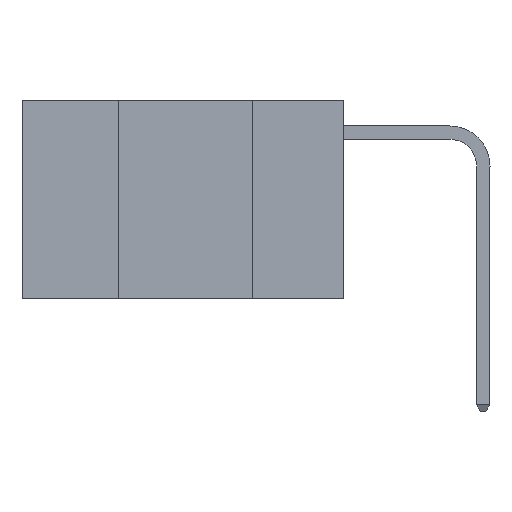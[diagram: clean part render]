
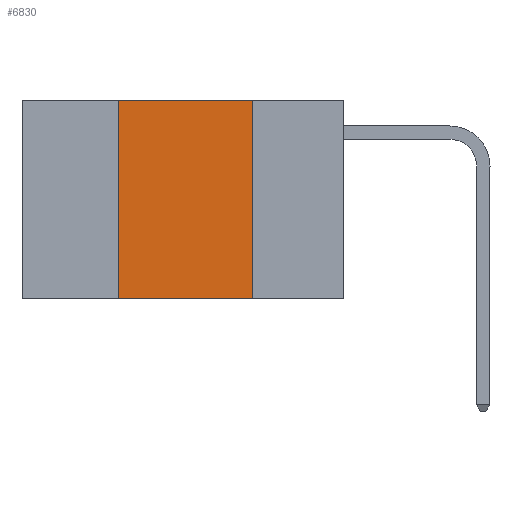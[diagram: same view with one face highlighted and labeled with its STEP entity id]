
A CAD part, left-side view. The second image highlights one B-rep face of the part: STEP entity #6830.
In plain terms, the highlighted planar face has unit normal (-1, 0, 0).
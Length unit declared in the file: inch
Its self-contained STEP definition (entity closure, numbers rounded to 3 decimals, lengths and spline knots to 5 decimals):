
#177 = PLANE ( 'NONE',  #2435 ) ;
#369 = VERTEX_POINT ( 'NONE', #13710 ) ;
#544 = VECTOR ( 'NONE', #6239, 39.37008 ) ;
#710 = LINE ( 'NONE', #12599, #544 ) ;
#2435 = AXIS2_PLACEMENT_3D ( 'NONE', #6930, #13141, #13107 ) ;
#2529 = EDGE_LOOP ( 'NONE', ( #4558, #4366, #9722, #13300 ) ) ;
#2900 = VECTOR ( 'NONE', #13719, 39.37008 ) ;
#3080 = EDGE_CURVE ( 'NONE', #9470, #10870, #3262, .T. ) ;
#3173 = VECTOR ( 'NONE', #10405, 39.37008 ) ;
#3262 = LINE ( 'NONE', #10726, #3173 ) ;
#4156 = LINE ( 'NONE', #7508, #2900 ) ;
#4281 = CARTESIAN_POINT ( 'NONE',  ( 0., 0.17, 0. ) ) ;
#4366 = ORIENTED_EDGE ( 'NONE', *, *, #11066, .F. ) ;
#4558 = ORIENTED_EDGE ( 'NONE', *, *, #10355, .F. ) ;
#4581 = DIRECTION ( 'NONE',  ( 0., 0., 1. ) ) ;
#5037 = CARTESIAN_POINT ( 'NONE',  ( 0., 0.42, 0. ) ) ;
#5210 = EDGE_CURVE ( 'NONE', #9470, #369, #12428, .T. ) ;
#6239 = DIRECTION ( 'NONE',  ( 0., 0., -1. ) ) ;
#6830 = ADVANCED_FACE ( 'NONE', ( #8555 ), #177, .F. ) ;
#6930 = CARTESIAN_POINT ( 'NONE',  ( 0., 0.6, 0. ) ) ;
#7508 = CARTESIAN_POINT ( 'NONE',  ( 0., 0.6, 0. ) ) ;
#8555 = FACE_OUTER_BOUND ( 'NONE', #2529, .T. ) ;
#9470 = VERTEX_POINT ( 'NONE', #12222 ) ;
#9722 = ORIENTED_EDGE ( 'NONE', *, *, #5210, .F. ) ;
#10355 = EDGE_CURVE ( 'NONE', #10476, #10870, #710, .T. ) ;
#10405 = DIRECTION ( 'NONE',  ( 0., -1., 0. ) ) ;
#10476 = VERTEX_POINT ( 'NONE', #4281 ) ;
#10726 = CARTESIAN_POINT ( 'NONE',  ( 0., 0.6, -0.37 ) ) ;
#10870 = VERTEX_POINT ( 'NONE', #13394 ) ;
#11066 = EDGE_CURVE ( 'NONE', #369, #10476, #4156, .T. ) ;
#11829 = VECTOR ( 'NONE', #4581, 39.37008 ) ;
#12222 = CARTESIAN_POINT ( 'NONE',  ( 0., 0.42, -0.37 ) ) ;
#12428 = LINE ( 'NONE', #5037, #11829 ) ;
#12599 = CARTESIAN_POINT ( 'NONE',  ( 0., 0.17, 0. ) ) ;
#13107 = DIRECTION ( 'NONE',  ( 0., 0., -1. ) ) ;
#13141 = DIRECTION ( 'NONE',  ( 1., 0., 0. ) ) ;
#13300 = ORIENTED_EDGE ( 'NONE', *, *, #3080, .T. ) ;
#13394 = CARTESIAN_POINT ( 'NONE',  ( 0., 0.17, -0.37 ) ) ;
#13710 = CARTESIAN_POINT ( 'NONE',  ( 0., 0.42, 0. ) ) ;
#13719 = DIRECTION ( 'NONE',  ( 0., -1., 0. ) ) ;
